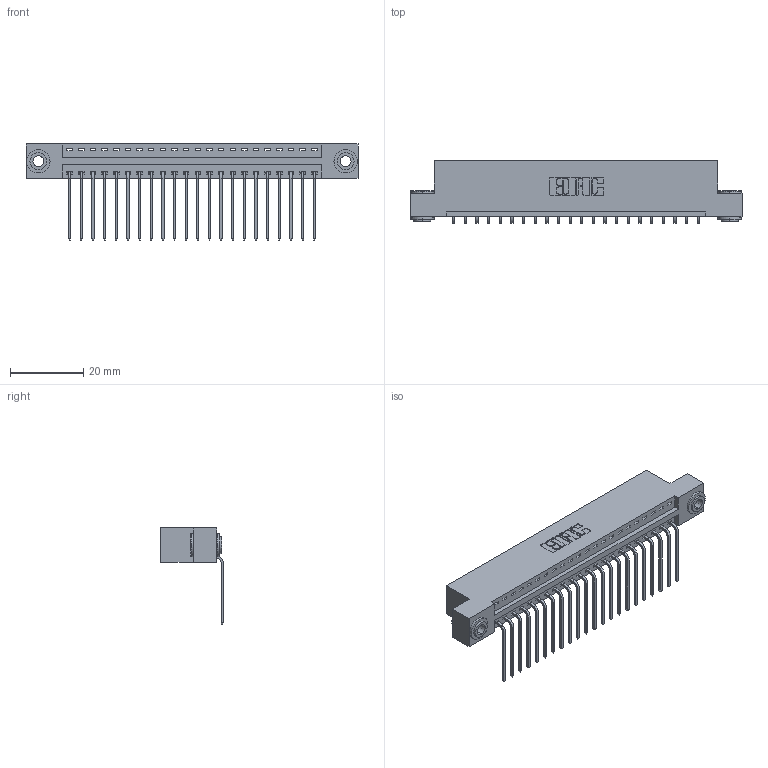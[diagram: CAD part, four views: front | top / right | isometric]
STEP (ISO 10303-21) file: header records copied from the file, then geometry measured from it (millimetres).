
FILE_DESCRIPTION (( 'STEP AP203' ), '1' );
FILE_NAME ('396-022-559-103.STEP', '2019-10-31T21:06:11', ( '' ), ( '' ), 'SwSTEP 2.0', 'SolidWorks 2016', '' );
FILE_SCHEMA (( 'CONFIG_CONTROL_DESIGN' ));
Length unit declared in the file: inch
Products named in the file (4): 346 Part_Flush Mounting Lugs - 0.156 Dia-TH; 345-292-001_558 559 Tail - 1; 345-250-002_345-250-002-102; 396-022-559-103
Assembly tree (25 placements, depth 2):
  396-022-559-103
    346 Part_Flush Mounting Lugs - 0.156 Dia-TH
    345-292-001_558 559 Tail - 1  x22
    345-250-002_345-250-002-102  x2
Bounding box: 90.42 x 17.08 x 26.16 mm (x, y, z)
Volume: 8610.5 mm3; surface area: 11202.6 mm2
Topology: 25 solids, 25 shells, 1480 faces, 4409 edges, 2906 vertices
Faces by surface type: plane 1010, cylinder 462, cone 8
Entity records: 17080 total; most frequent: CARTESIAN_POINT 2913, ORIENTED_EDGE 2862, DIRECTION 2625, EDGE_CURVE 1431, LINE 1187, VECTOR 1187, VERTEX_POINT 950, AXIS2_PLACEMENT_3D 719
